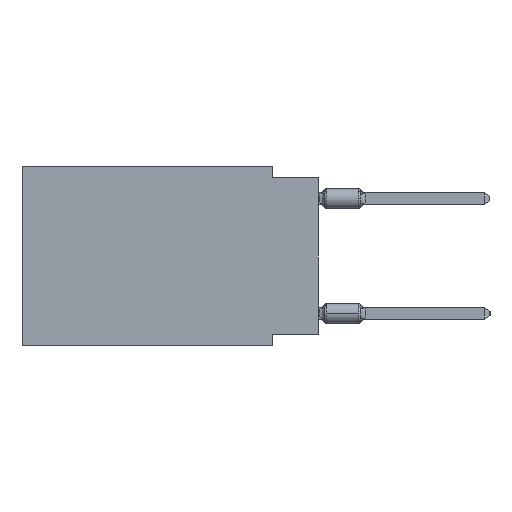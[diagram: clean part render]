
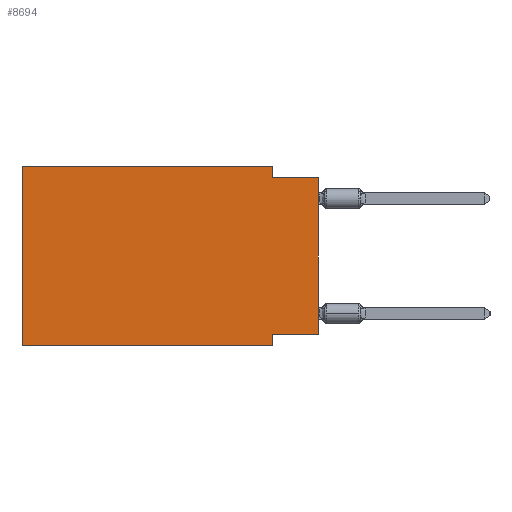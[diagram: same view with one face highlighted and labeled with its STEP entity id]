
A CAD part, left-side view. The second image highlights one B-rep face of the part: STEP entity #8694.
In plain terms, the highlighted planar face has unit normal (-1, 0, 0).
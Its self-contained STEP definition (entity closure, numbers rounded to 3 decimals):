
#1083 = EDGE_CURVE ( 'NONE', #22153, #38321, #13055, .T. ) ;
#2727 = CARTESIAN_POINT ( 'NONE',  ( 0., 2.54, 0. ) ) ;
#2858 = DIRECTION ( 'NONE',  ( 1., 0., 0. ) ) ;
#2963 = LINE ( 'NONE', #27379, #30291 ) ;
#5204 = EDGE_CURVE ( 'NONE', #24027, #31313, #2963, .T. ) ;
#6346 = VECTOR ( 'NONE', #10245, 1000. ) ;
#6707 = VECTOR ( 'NONE', #22814, 1000. ) ;
#6998 = AXIS2_PLACEMENT_3D ( 'NONE', #29871, #2858, #8673 ) ;
#7459 = CARTESIAN_POINT ( 'NONE',  ( 0., 0., -9.271 ) ) ;
#7539 = CARTESIAN_POINT ( 'NONE',  ( 0., 16.383, 0. ) ) ;
#8673 = DIRECTION ( 'NONE',  ( 0., 0., -1. ) ) ;
#8694 = ADVANCED_FACE ( 'NONE', ( #17670 ), #18444, .F. ) ;
#9160 = DIRECTION ( 'NONE',  ( 0., 0., 1. ) ) ;
#9277 = ORIENTED_EDGE ( 'NONE', *, *, #5204, .F. ) ;
#9839 = EDGE_CURVE ( 'NONE', #31313, #15394, #38037, .T. ) ;
#9931 = CARTESIAN_POINT ( 'NONE',  ( 0., 0., -0.635 ) ) ;
#10245 = DIRECTION ( 'NONE',  ( 0., 0., -1. ) ) ;
#10353 = CARTESIAN_POINT ( 'NONE',  ( 0., 2.54, -9.906 ) ) ;
#10383 = CARTESIAN_POINT ( 'NONE',  ( 0., 16.383, 0. ) ) ;
#10419 = VERTEX_POINT ( 'NONE', #38770 ) ;
#10586 = EDGE_CURVE ( 'NONE', #10419, #18931, #31470, .T. ) ;
#10673 = ORIENTED_EDGE ( 'NONE', *, *, #10586, .F. ) ;
#10714 = ORIENTED_EDGE ( 'NONE', *, *, #1083, .F. ) ;
#11592 = VECTOR ( 'NONE', #25452, 1000. ) ;
#11917 = VECTOR ( 'NONE', #26735, 1000. ) ;
#12212 = VECTOR ( 'NONE', #32746, 1000. ) ;
#13055 = LINE ( 'NONE', #31486, #6346 ) ;
#13909 = LINE ( 'NONE', #29125, #12212 ) ;
#14338 = LINE ( 'NONE', #2727, #24034 ) ;
#15394 = VERTEX_POINT ( 'NONE', #26249 ) ;
#17124 = CARTESIAN_POINT ( 'NONE',  ( 0., 16.383, -9.906 ) ) ;
#17210 = LINE ( 'NONE', #20196, #6707 ) ;
#17670 = FACE_OUTER_BOUND ( 'NONE', #20967, .T. ) ;
#17779 = EDGE_CURVE ( 'NONE', #33526, #18931, #13909, .T. ) ;
#18444 = PLANE ( 'NONE',  #6998 ) ;
#18931 = VERTEX_POINT ( 'NONE', #9931 ) ;
#19082 = EDGE_CURVE ( 'NONE', #24027, #38321, #29927, .T. ) ;
#19208 = VECTOR ( 'NONE', #22400, 1000. ) ;
#20196 = CARTESIAN_POINT ( 'NONE',  ( 0., 0., -9.271 ) ) ;
#20967 = EDGE_LOOP ( 'NONE', ( #27806, #10673, #32235, #21908, #9277, #25770, #10714, #32876 ) ) ;
#21908 = ORIENTED_EDGE ( 'NONE', *, *, #9839, .F. ) ;
#22153 = VERTEX_POINT ( 'NONE', #23430 ) ;
#22400 = DIRECTION ( 'NONE',  ( 0., -1., 0. ) ) ;
#22814 = DIRECTION ( 'NONE',  ( 0., 1., 0. ) ) ;
#23430 = CARTESIAN_POINT ( 'NONE',  ( 0., 2.54, -9.271 ) ) ;
#24027 = VERTEX_POINT ( 'NONE', #27212 ) ;
#24034 = VECTOR ( 'NONE', #29557, 1000. ) ;
#25452 = DIRECTION ( 'NONE',  ( 0., -1., 0. ) ) ;
#25770 = ORIENTED_EDGE ( 'NONE', *, *, #19082, .T. ) ;
#26249 = CARTESIAN_POINT ( 'NONE',  ( 0., 2.54, 0. ) ) ;
#26735 = DIRECTION ( 'NONE',  ( 0., -1., 0. ) ) ;
#27212 = CARTESIAN_POINT ( 'NONE',  ( 0., 16.383, -9.906 ) ) ;
#27379 = CARTESIAN_POINT ( 'NONE',  ( 0., 16.383, 0. ) ) ;
#27806 = ORIENTED_EDGE ( 'NONE', *, *, #17779, .T. ) ;
#28453 = CARTESIAN_POINT ( 'NONE',  ( 0., 0., -0.635 ) ) ;
#29125 = CARTESIAN_POINT ( 'NONE',  ( 0., 0., 0. ) ) ;
#29557 = DIRECTION ( 'NONE',  ( 0., 0., -1. ) ) ;
#29871 = CARTESIAN_POINT ( 'NONE',  ( 0., 16.383, 0. ) ) ;
#29927 = LINE ( 'NONE', #17124, #11917 ) ;
#30291 = VECTOR ( 'NONE', #9160, 1000. ) ;
#30410 = EDGE_CURVE ( 'NONE', #33526, #22153, #17210, .T. ) ;
#31313 = VERTEX_POINT ( 'NONE', #7539 ) ;
#31407 = EDGE_CURVE ( 'NONE', #15394, #10419, #14338, .T. ) ;
#31470 = LINE ( 'NONE', #28453, #11592 ) ;
#31486 = CARTESIAN_POINT ( 'NONE',  ( 0., 2.54, -9.906 ) ) ;
#32235 = ORIENTED_EDGE ( 'NONE', *, *, #31407, .F. ) ;
#32746 = DIRECTION ( 'NONE',  ( 0., 0., 1. ) ) ;
#32876 = ORIENTED_EDGE ( 'NONE', *, *, #30410, .F. ) ;
#33526 = VERTEX_POINT ( 'NONE', #7459 ) ;
#38037 = LINE ( 'NONE', #10383, #19208 ) ;
#38321 = VERTEX_POINT ( 'NONE', #10353 ) ;
#38770 = CARTESIAN_POINT ( 'NONE',  ( 0., 2.54, -0.635 ) ) ;
